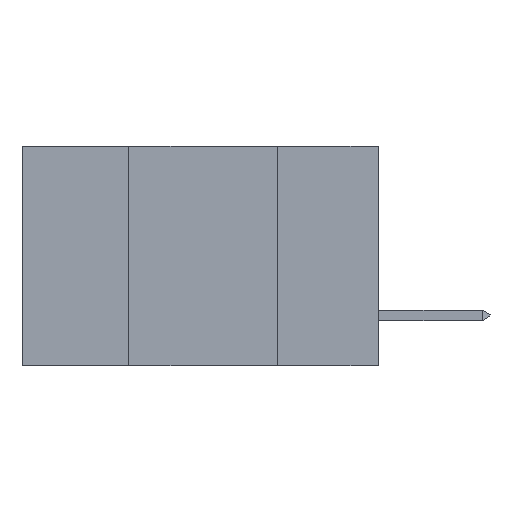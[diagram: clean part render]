
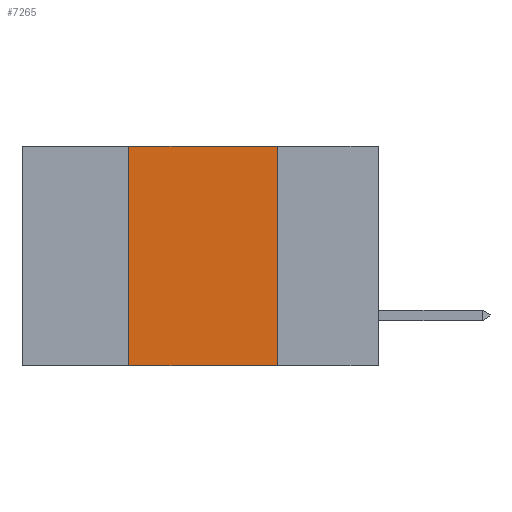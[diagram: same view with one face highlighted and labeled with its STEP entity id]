
A CAD part, left-side view. The second image highlights one B-rep face of the part: STEP entity #7265.
In plain terms, the highlighted planar face has unit normal (-1, 0, 0).
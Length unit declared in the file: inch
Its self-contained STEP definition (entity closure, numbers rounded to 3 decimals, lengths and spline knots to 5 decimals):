
#95 = CARTESIAN_POINT ( 'NONE',  ( 0., 0.42, -0.37 ) ) ;
#530 = VERTEX_POINT ( 'NONE', #9630 ) ;
#610 = ORIENTED_EDGE ( 'NONE', *, *, #8426, .F. ) ;
#667 = DIRECTION ( 'NONE',  ( 0., 0., -1. ) ) ;
#733 = AXIS2_PLACEMENT_3D ( 'NONE', #5554, #8755, #6284 ) ;
#1070 = DIRECTION ( 'NONE',  ( 0., -1., 0. ) ) ;
#1813 = CARTESIAN_POINT ( 'NONE',  ( 0., 0.42, 0. ) ) ;
#2112 = CARTESIAN_POINT ( 'NONE',  ( 0., 0.17, -0.37 ) ) ;
#2113 = ORIENTED_EDGE ( 'NONE', *, *, #7118, .F. ) ;
#2348 = FACE_OUTER_BOUND ( 'NONE', #9334, .T. ) ;
#2744 = VECTOR ( 'NONE', #4673, 39.37008 ) ;
#2982 = DIRECTION ( 'NONE',  ( 0., -1., 0. ) ) ;
#3267 = ORIENTED_EDGE ( 'NONE', *, *, #5440, .T. ) ;
#3417 = LINE ( 'NONE', #8208, #8876 ) ;
#3832 = LINE ( 'NONE', #6806, #9041 ) ;
#4082 = PLANE ( 'NONE',  #733 ) ;
#4130 = VERTEX_POINT ( 'NONE', #1813 ) ;
#4673 = DIRECTION ( 'NONE',  ( 0., 0., 1. ) ) ;
#5244 = VERTEX_POINT ( 'NONE', #95 ) ;
#5304 = LINE ( 'NONE', #5507, #2744 ) ;
#5440 = EDGE_CURVE ( 'NONE', #5244, #530, #3417, .T. ) ;
#5507 = CARTESIAN_POINT ( 'NONE',  ( 0., 0.42, -0.37 ) ) ;
#5554 = CARTESIAN_POINT ( 'NONE',  ( 0., 0.6, 0. ) ) ;
#6284 = DIRECTION ( 'NONE',  ( 0., 0., -1. ) ) ;
#6311 = EDGE_CURVE ( 'NONE', #9226, #530, #9256, .T. ) ;
#6806 = CARTESIAN_POINT ( 'NONE',  ( 0., 0.6, 0. ) ) ;
#7118 = EDGE_CURVE ( 'NONE', #4130, #9226, #3832, .T. ) ;
#7265 = ADVANCED_FACE ( 'NONE', ( #2348 ), #4082, .F. ) ;
#8205 = VECTOR ( 'NONE', #667, 39.37008 ) ;
#8208 = CARTESIAN_POINT ( 'NONE',  ( 0., 0.6, -0.37 ) ) ;
#8426 = EDGE_CURVE ( 'NONE', #5244, #4130, #5304, .T. ) ;
#8612 = CARTESIAN_POINT ( 'NONE',  ( 0., 0.17, 0. ) ) ;
#8753 = ORIENTED_EDGE ( 'NONE', *, *, #6311, .F. ) ;
#8755 = DIRECTION ( 'NONE',  ( 1., 0., 0. ) ) ;
#8876 = VECTOR ( 'NONE', #1070, 39.37008 ) ;
#9041 = VECTOR ( 'NONE', #2982, 39.37008 ) ;
#9226 = VERTEX_POINT ( 'NONE', #8612 ) ;
#9256 = LINE ( 'NONE', #2112, #8205 ) ;
#9334 = EDGE_LOOP ( 'NONE', ( #8753, #2113, #610, #3267 ) ) ;
#9630 = CARTESIAN_POINT ( 'NONE',  ( 0., 0.17, -0.37 ) ) ;
